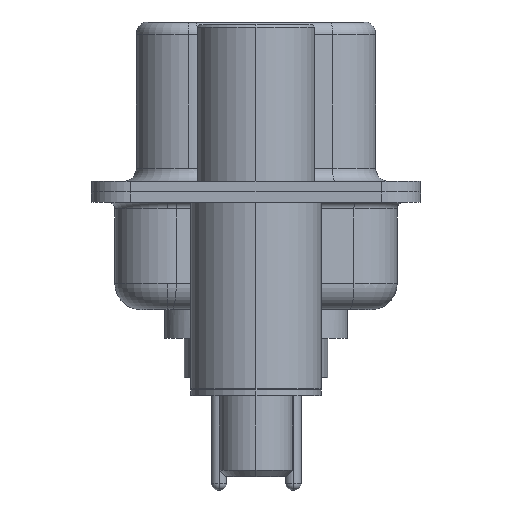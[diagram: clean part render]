
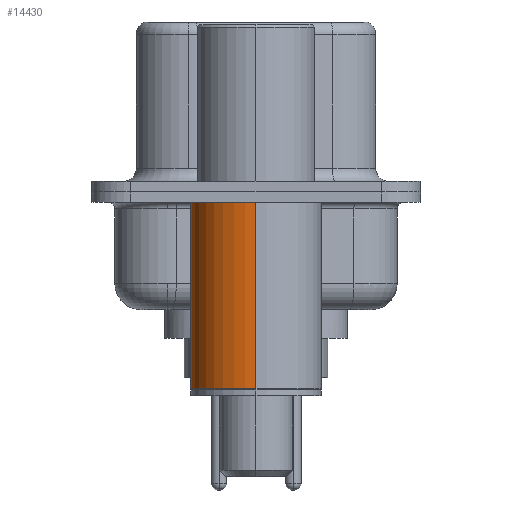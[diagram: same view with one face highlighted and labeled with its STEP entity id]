
A CAD part, left-side view. The second image highlights one B-rep face of the part: STEP entity #14430.
In plain terms, the highlighted cylindrical face has radius 2.5 mm (diameter 5 mm), a partial arc.
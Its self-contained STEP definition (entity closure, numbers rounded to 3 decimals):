
#208 = DIRECTION ( 'NONE',  ( 0., 0., 1. ) ) ;
#229 = EDGE_CURVE ( 'NONE', #21279, #16563, #5891, .T. ) ;
#421 = EDGE_CURVE ( 'NONE', #4030, #16563, #3800, .T. ) ;
#1260 = CARTESIAN_POINT ( 'NONE',  ( -2.5, 0., -7.525 ) ) ;
#1269 = CARTESIAN_POINT ( 'NONE',  ( 0., 0., -0.4 ) ) ;
#1337 = AXIS2_PLACEMENT_3D ( 'NONE', #1269, #208, #13118 ) ;
#2213 = EDGE_CURVE ( 'NONE', #11108, #4030, #9002, .T. ) ;
#2554 = ORIENTED_EDGE ( 'NONE', *, *, #421, .T. ) ;
#3434 = CARTESIAN_POINT ( 'NONE',  ( 2.5, 0., 0.581 ) ) ;
#3618 = ORIENTED_EDGE ( 'NONE', *, *, #229, .F. ) ;
#3800 = LINE ( 'NONE', #17396, #22067 ) ;
#4030 = VERTEX_POINT ( 'NONE', #1260 ) ;
#4113 = CARTESIAN_POINT ( 'NONE',  ( -2.5, 0., -0.4 ) ) ;
#4258 = FACE_OUTER_BOUND ( 'NONE', #20566, .T. ) ;
#5057 = DIRECTION ( 'NONE',  ( 1., 0., 0. ) ) ;
#5322 = DIRECTION ( 'NONE',  ( 1., 0., 0. ) ) ;
#5410 = CARTESIAN_POINT ( 'NONE',  ( 0., 0., -7.525 ) ) ;
#5509 = DIRECTION ( 'NONE',  ( 0., 0., 1. ) ) ;
#5891 = CIRCLE ( 'NONE', #1337, 2.5 ) ;
#7046 = DIRECTION ( 'NONE',  ( 0., 0., 1. ) ) ;
#7667 = AXIS2_PLACEMENT_3D ( 'NONE', #17761, #7046, #5322 ) ;
#8914 = DIRECTION ( 'NONE',  ( 0., 0., 1. ) ) ;
#9002 = CIRCLE ( 'NONE', #22685, 2.5 ) ;
#11108 = VERTEX_POINT ( 'NONE', #16869 ) ;
#11293 = ORIENTED_EDGE ( 'NONE', *, *, #2213, .T. ) ;
#11917 = CARTESIAN_POINT ( 'NONE',  ( 2.5, 0., -0.4 ) ) ;
#13118 = DIRECTION ( 'NONE',  ( 1., 0., 0. ) ) ;
#13157 = CYLINDRICAL_SURFACE ( 'NONE', #7667, 2.5 ) ;
#14430 = ADVANCED_FACE ( 'NONE', ( #4258 ), #13157, .T. ) ;
#15306 = EDGE_CURVE ( 'NONE', #11108, #21279, #21411, .T. ) ;
#16563 = VERTEX_POINT ( 'NONE', #4113 ) ;
#16692 = VECTOR ( 'NONE', #17501, 1000. ) ;
#16869 = CARTESIAN_POINT ( 'NONE',  ( 2.5, 0., -7.525 ) ) ;
#17396 = CARTESIAN_POINT ( 'NONE',  ( -2.5, 0., 0.581 ) ) ;
#17501 = DIRECTION ( 'NONE',  ( 0., 0., 1. ) ) ;
#17761 = CARTESIAN_POINT ( 'NONE',  ( 0., 0., 0.581 ) ) ;
#18062 = ORIENTED_EDGE ( 'NONE', *, *, #15306, .F. ) ;
#20566 = EDGE_LOOP ( 'NONE', ( #11293, #2554, #3618, #18062 ) ) ;
#21279 = VERTEX_POINT ( 'NONE', #11917 ) ;
#21411 = LINE ( 'NONE', #3434, #16692 ) ;
#22067 = VECTOR ( 'NONE', #8914, 1000. ) ;
#22685 = AXIS2_PLACEMENT_3D ( 'NONE', #5410, #5509, #5057 ) ;
